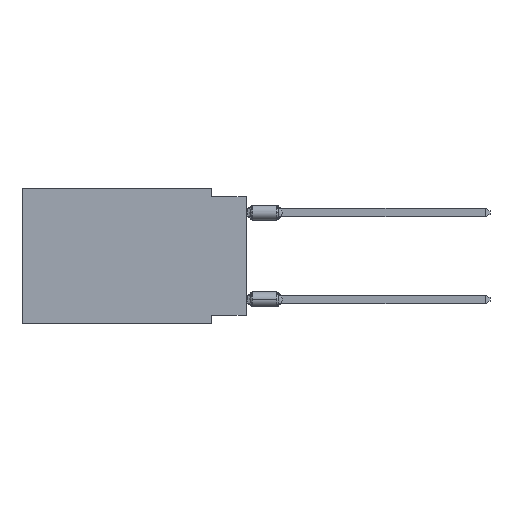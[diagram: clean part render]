
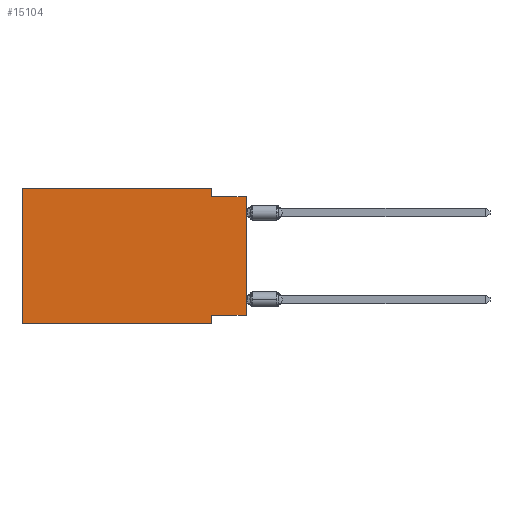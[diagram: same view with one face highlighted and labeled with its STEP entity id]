
A CAD part, left-side view. The second image highlights one B-rep face of the part: STEP entity #15104.
In plain terms, the highlighted planar face has unit normal (-1, 0, 0).
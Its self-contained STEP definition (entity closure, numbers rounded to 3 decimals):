
#1228 = CARTESIAN_POINT ( 'NONE',  ( 0., 2.54, 0. ) ) ;
#1721 = EDGE_CURVE ( 'NONE', #11905, #16808, #3491, .T. ) ;
#1965 = VECTOR ( 'NONE', #2144, 1000. ) ;
#2053 = PLANE ( 'NONE',  #31097 ) ;
#2144 = DIRECTION ( 'NONE',  ( 0., 0., 1. ) ) ;
#2808 = LINE ( 'NONE', #24573, #17310 ) ;
#3122 = LINE ( 'NONE', #27090, #19316 ) ;
#3491 = LINE ( 'NONE', #11054, #28768 ) ;
#3532 = EDGE_CURVE ( 'NONE', #24854, #18257, #2808, .T. ) ;
#3897 = EDGE_CURVE ( 'NONE', #27199, #24854, #18987, .T. ) ;
#4461 = ORIENTED_EDGE ( 'NONE', *, *, #25714, .T. ) ;
#4553 = ORIENTED_EDGE ( 'NONE', *, *, #3897, .F. ) ;
#5312 = LINE ( 'NONE', #14917, #25960 ) ;
#5336 = DIRECTION ( 'NONE',  ( 0., -1., 0. ) ) ;
#6068 = ORIENTED_EDGE ( 'NONE', *, *, #6639, .T. ) ;
#6299 = ORIENTED_EDGE ( 'NONE', *, *, #3532, .F. ) ;
#6528 = ORIENTED_EDGE ( 'NONE', *, *, #14205, .F. ) ;
#6639 = EDGE_CURVE ( 'NONE', #22065, #16808, #3122, .T. ) ;
#6697 = DIRECTION ( 'NONE',  ( 0., 0., -1. ) ) ;
#6843 = CARTESIAN_POINT ( 'NONE',  ( 0., 2.54, -0.635 ) ) ;
#8134 = EDGE_CURVE ( 'NONE', #22065, #8742, #19021, .T. ) ;
#8742 = VERTEX_POINT ( 'NONE', #19137 ) ;
#9453 = CARTESIAN_POINT ( 'NONE',  ( 0., 16.383, 0. ) ) ;
#11054 = CARTESIAN_POINT ( 'NONE',  ( 0., 0., -0.635 ) ) ;
#11905 = VERTEX_POINT ( 'NONE', #6843 ) ;
#12764 = VERTEX_POINT ( 'NONE', #25964 ) ;
#13039 = DIRECTION ( 'NONE',  ( 0., 0., 1. ) ) ;
#13046 = LINE ( 'NONE', #1228, #29543 ) ;
#13863 = ORIENTED_EDGE ( 'NONE', *, *, #1721, .F. ) ;
#14205 = EDGE_CURVE ( 'NONE', #18257, #11905, #13046, .T. ) ;
#14917 = CARTESIAN_POINT ( 'NONE',  ( 0., 2.54, -9.906 ) ) ;
#15078 = DIRECTION ( 'NONE',  ( 0., 0., -1. ) ) ;
#15104 = ADVANCED_FACE ( 'NONE', ( #30600 ), #2053, .F. ) ;
#15141 = ORIENTED_EDGE ( 'NONE', *, *, #21344, .F. ) ;
#16176 = CARTESIAN_POINT ( 'NONE',  ( 0., 2.54, 0. ) ) ;
#16646 = CARTESIAN_POINT ( 'NONE',  ( 0., 16.383, 0. ) ) ;
#16808 = VERTEX_POINT ( 'NONE', #29136 ) ;
#16839 = DIRECTION ( 'NONE',  ( 0., 0., -1. ) ) ;
#17310 = VECTOR ( 'NONE', #5336, 1000. ) ;
#18257 = VERTEX_POINT ( 'NONE', #16176 ) ;
#18987 = LINE ( 'NONE', #20902, #1965 ) ;
#19021 = LINE ( 'NONE', #30573, #23928 ) ;
#19137 = CARTESIAN_POINT ( 'NONE',  ( 0., 2.54, -9.271 ) ) ;
#19316 = VECTOR ( 'NONE', #13039, 1000. ) ;
#19988 = LINE ( 'NONE', #27254, #20502 ) ;
#20502 = VECTOR ( 'NONE', #29472, 1000. ) ;
#20902 = CARTESIAN_POINT ( 'NONE',  ( 0., 16.383, 0. ) ) ;
#21239 = DIRECTION ( 'NONE',  ( 0., 1., 0. ) ) ;
#21344 = EDGE_CURVE ( 'NONE', #8742, #12764, #5312, .T. ) ;
#21425 = ORIENTED_EDGE ( 'NONE', *, *, #8134, .F. ) ;
#22065 = VERTEX_POINT ( 'NONE', #26057 ) ;
#23928 = VECTOR ( 'NONE', #21239, 1000. ) ;
#24573 = CARTESIAN_POINT ( 'NONE',  ( 0., 16.383, 0. ) ) ;
#24854 = VERTEX_POINT ( 'NONE', #16646 ) ;
#25714 = EDGE_CURVE ( 'NONE', #27199, #12764, #19988, .T. ) ;
#25960 = VECTOR ( 'NONE', #15078, 1000. ) ;
#25964 = CARTESIAN_POINT ( 'NONE',  ( 0., 2.54, -9.906 ) ) ;
#26012 = DIRECTION ( 'NONE',  ( 1., 0., 0. ) ) ;
#26057 = CARTESIAN_POINT ( 'NONE',  ( 0., 0., -9.271 ) ) ;
#27090 = CARTESIAN_POINT ( 'NONE',  ( 0., 0., 0. ) ) ;
#27199 = VERTEX_POINT ( 'NONE', #28084 ) ;
#27254 = CARTESIAN_POINT ( 'NONE',  ( 0., 16.383, -9.906 ) ) ;
#28084 = CARTESIAN_POINT ( 'NONE',  ( 0., 16.383, -9.906 ) ) ;
#28768 = VECTOR ( 'NONE', #30297, 1000. ) ;
#28965 = EDGE_LOOP ( 'NONE', ( #6068, #13863, #6528, #6299, #4553, #4461, #15141, #21425 ) ) ;
#29136 = CARTESIAN_POINT ( 'NONE',  ( 0., 0., -0.635 ) ) ;
#29472 = DIRECTION ( 'NONE',  ( 0., -1., 0. ) ) ;
#29543 = VECTOR ( 'NONE', #6697, 1000. ) ;
#30297 = DIRECTION ( 'NONE',  ( 0., -1., 0. ) ) ;
#30573 = CARTESIAN_POINT ( 'NONE',  ( 0., 0., -9.271 ) ) ;
#30600 = FACE_OUTER_BOUND ( 'NONE', #28965, .T. ) ;
#31097 = AXIS2_PLACEMENT_3D ( 'NONE', #9453, #26012, #16839 ) ;
